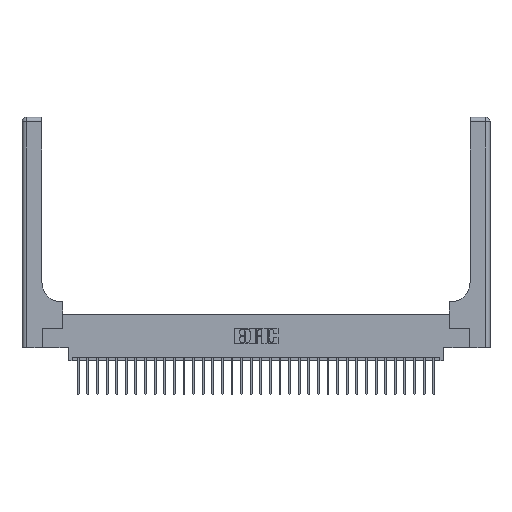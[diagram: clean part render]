
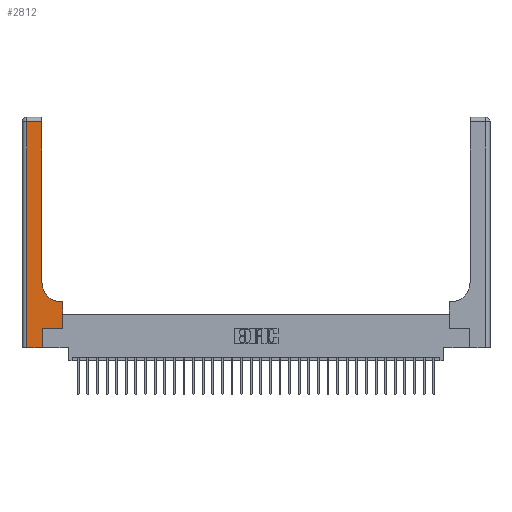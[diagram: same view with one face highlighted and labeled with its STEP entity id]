
A CAD part, top view. The second image highlights one B-rep face of the part: STEP entity #2812.
In plain terms, the highlighted planar face has unit normal (0, 0, 1).
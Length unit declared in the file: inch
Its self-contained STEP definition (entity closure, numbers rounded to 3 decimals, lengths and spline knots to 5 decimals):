
#20 = VECTOR ( 'NONE', #29614, 39.37008 ) ;
#2310 = VERTEX_POINT ( 'NONE', #30177 ) ;
#2587 = DIRECTION ( 'NONE',  ( 0., 1., 0. ) ) ;
#2812 = ADVANCED_FACE ( 'NONE', ( #30512 ), #4491, .F. ) ;
#3230 = LINE ( 'NONE', #20074, #26755 ) ;
#3736 = ORIENTED_EDGE ( 'NONE', *, *, #20034, .T. ) ;
#3869 = DIRECTION ( 'NONE',  ( 1., 0., 0. ) ) ;
#4491 = PLANE ( 'NONE',  #22593 ) ;
#4539 = CARTESIAN_POINT ( 'NONE',  ( 0.265, 0., 0.37 ) ) ;
#5097 = CARTESIAN_POINT ( 'NONE',  ( 0.528, 0.6, 0.37 ) ) ;
#5697 = EDGE_CURVE ( 'NONE', #7979, #13213, #25094, .T. ) ;
#5839 = CARTESIAN_POINT ( 'NONE',  ( 0.26, 2.94, 0.37 ) ) ;
#5950 = LINE ( 'NONE', #13067, #9742 ) ;
#6154 = VERTEX_POINT ( 'NONE', #5097 ) ;
#6728 = EDGE_CURVE ( 'NONE', #20819, #15744, #18083, .T. ) ;
#6876 = CARTESIAN_POINT ( 'NONE',  ( 0.265, 0.25, 0.37 ) ) ;
#7409 = EDGE_LOOP ( 'NONE', ( #20447, #30145, #10696, #10690, #13622, #12721, #3736, #18221, #19105 ) ) ;
#7979 = VERTEX_POINT ( 'NONE', #9272 ) ;
#8268 = DIRECTION ( 'NONE',  ( 0., -1., 0. ) ) ;
#8908 = DIRECTION ( 'NONE',  ( 0., 1., 0. ) ) ;
#9272 = CARTESIAN_POINT ( 'NONE',  ( 0.51, 0.6, 0.37 ) ) ;
#9338 = LINE ( 'NONE', #9484, #11698 ) ;
#9392 = DIRECTION ( 'NONE',  ( 0., 0., -1. ) ) ;
#9484 = CARTESIAN_POINT ( 'NONE',  ( 0., 2.94, 0.37 ) ) ;
#9693 = VECTOR ( 'NONE', #2587, 39.37008 ) ;
#9742 = VECTOR ( 'NONE', #25022, 39.37008 ) ;
#10690 = ORIENTED_EDGE ( 'NONE', *, *, #30094, .T. ) ;
#10696 = ORIENTED_EDGE ( 'NONE', *, *, #24702, .T. ) ;
#11698 = VECTOR ( 'NONE', #12153, 39.37008 ) ;
#12153 = DIRECTION ( 'NONE',  ( -1., 0., 0. ) ) ;
#12721 = ORIENTED_EDGE ( 'NONE', *, *, #6728, .T. ) ;
#13067 = CARTESIAN_POINT ( 'NONE',  ( 0.26, 0.6, 0.37 ) ) ;
#13213 = VERTEX_POINT ( 'NONE', #25125 ) ;
#13251 = VECTOR ( 'NONE', #8908, 39.37008 ) ;
#13622 = ORIENTED_EDGE ( 'NONE', *, *, #30285, .T. ) ;
#14062 = CARTESIAN_POINT ( 'NONE',  ( 0.265, 0., 0.37 ) ) ;
#14270 = VECTOR ( 'NONE', #26506, 39.37008 ) ;
#14733 = DIRECTION ( 'NONE',  ( 0., 0., -1. ) ) ;
#15280 = VECTOR ( 'NONE', #25493, 39.37008 ) ;
#15744 = VERTEX_POINT ( 'NONE', #16227 ) ;
#15894 = CARTESIAN_POINT ( 'NONE',  ( 0., 0., 0.37 ) ) ;
#16003 = CARTESIAN_POINT ( 'NONE',  ( 0., 3., 0.37 ) ) ;
#16084 = AXIS2_PLACEMENT_3D ( 'NONE', #26701, #14733, #3869 ) ;
#16227 = CARTESIAN_POINT ( 'NONE',  ( 0.528, 0.25, 0.37 ) ) ;
#17703 = VERTEX_POINT ( 'NONE', #4539 ) ;
#18083 = LINE ( 'NONE', #29922, #20 ) ;
#18221 = ORIENTED_EDGE ( 'NONE', *, *, #30108, .T. ) ;
#18824 = LINE ( 'NONE', #24013, #9693 ) ;
#19105 = ORIENTED_EDGE ( 'NONE', *, *, #5697, .T. ) ;
#20034 = EDGE_CURVE ( 'NONE', #15744, #6154, #18824, .T. ) ;
#20074 = CARTESIAN_POINT ( 'NONE',  ( 0.06, 3., 0.37 ) ) ;
#20447 = ORIENTED_EDGE ( 'NONE', *, *, #28134, .T. ) ;
#20819 = VERTEX_POINT ( 'NONE', #6876 ) ;
#21309 = CARTESIAN_POINT ( 'NONE',  ( 0.26, 3., 0.37 ) ) ;
#22593 = AXIS2_PLACEMENT_3D ( 'NONE', #16003, #9392, #25591 ) ;
#24013 = CARTESIAN_POINT ( 'NONE',  ( 0.528, 0.25, 0.37 ) ) ;
#24371 = CARTESIAN_POINT ( 'NONE',  ( 0.06, 2.94, 0.37 ) ) ;
#24702 = EDGE_CURVE ( 'NONE', #26073, #2310, #3230, .T. ) ;
#25022 = DIRECTION ( 'NONE',  ( -1., 0., 0. ) ) ;
#25094 = CIRCLE ( 'NONE', #16084, 0.25 ) ;
#25125 = CARTESIAN_POINT ( 'NONE',  ( 0.26, 0.85, 0.37 ) ) ;
#25138 = VERTEX_POINT ( 'NONE', #5839 ) ;
#25366 = EDGE_CURVE ( 'NONE', #25138, #26073, #9338, .T. ) ;
#25493 = DIRECTION ( 'NONE',  ( 1., 0., 0. ) ) ;
#25591 = DIRECTION ( 'NONE',  ( -1., 0., 0. ) ) ;
#26073 = VERTEX_POINT ( 'NONE', #24371 ) ;
#26197 = LINE ( 'NONE', #14062, #14270 ) ;
#26506 = DIRECTION ( 'NONE',  ( 0., 1., 0. ) ) ;
#26701 = CARTESIAN_POINT ( 'NONE',  ( 0.51, 0.85, 0.37 ) ) ;
#26755 = VECTOR ( 'NONE', #8268, 39.37008 ) ;
#28134 = EDGE_CURVE ( 'NONE', #13213, #25138, #30647, .T. ) ;
#29614 = DIRECTION ( 'NONE',  ( 1., 0., 0. ) ) ;
#29922 = CARTESIAN_POINT ( 'NONE',  ( 0.265, 0.25, 0.37 ) ) ;
#29925 = LINE ( 'NONE', #15894, #15280 ) ;
#30094 = EDGE_CURVE ( 'NONE', #2310, #17703, #29925, .T. ) ;
#30108 = EDGE_CURVE ( 'NONE', #6154, #7979, #5950, .T. ) ;
#30145 = ORIENTED_EDGE ( 'NONE', *, *, #25366, .T. ) ;
#30177 = CARTESIAN_POINT ( 'NONE',  ( 0.06, 0., 0.37 ) ) ;
#30285 = EDGE_CURVE ( 'NONE', #17703, #20819, #26197, .T. ) ;
#30512 = FACE_OUTER_BOUND ( 'NONE', #7409, .T. ) ;
#30647 = LINE ( 'NONE', #21309, #13251 ) ;
